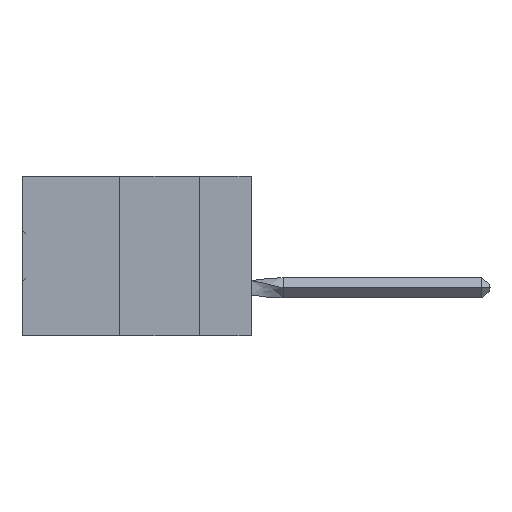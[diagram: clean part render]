
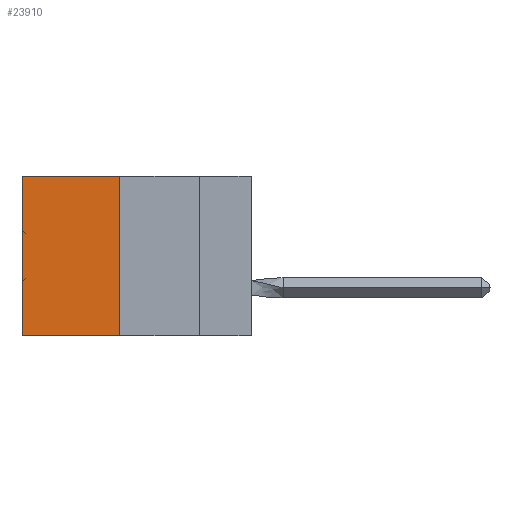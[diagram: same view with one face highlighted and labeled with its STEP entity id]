
A CAD part, left-side view. The second image highlights one B-rep face of the part: STEP entity #23910.
In plain terms, the highlighted planar face has unit normal (-1, 0, 0).
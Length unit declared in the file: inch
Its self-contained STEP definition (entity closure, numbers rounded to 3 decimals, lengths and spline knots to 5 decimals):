
#2695 = CARTESIAN_POINT ( 'NONE',  ( 0.305, 0.413, -0.5 ) ) ;
#3593 = DIRECTION ( 'NONE',  ( 0., 1., 0. ) ) ;
#4007 = CARTESIAN_POINT ( 'NONE',  ( 0.305, 0.413, 0. ) ) ;
#4763 = CARTESIAN_POINT ( 'NONE',  ( 0.305, 0.72, -0.5 ) ) ;
#7627 = CARTESIAN_POINT ( 'NONE',  ( 0.305, 0.413, -0.5 ) ) ;
#9942 = ORIENTED_EDGE ( 'NONE', *, *, #45272, .F. ) ;
#12156 = DIRECTION ( 'NONE',  ( 0., 1., 0. ) ) ;
#12192 = PLANE ( 'NONE',  #33463 ) ;
#13386 = VECTOR ( 'NONE', #12156, 39.37008 ) ;
#17268 = CARTESIAN_POINT ( 'NONE',  ( 0.305, 0.413, -0.5 ) ) ;
#17819 = VERTEX_POINT ( 'NONE', #25723 ) ;
#18130 = FACE_OUTER_BOUND ( 'NONE', #22927, .T. ) ;
#18788 = VECTOR ( 'NONE', #39322, 39.37008 ) ;
#19635 = VERTEX_POINT ( 'NONE', #52158 ) ;
#22927 = EDGE_LOOP ( 'NONE', ( #52261, #9942, #37800, #55808 ) ) ;
#23910 = ADVANCED_FACE ( 'NONE', ( #18130 ), #12192, .F. ) ;
#24987 = EDGE_CURVE ( 'NONE', #19635, #41648, #39858, .T. ) ;
#25723 = CARTESIAN_POINT ( 'NONE',  ( 0.305, 0.72, 0. ) ) ;
#33463 = AXIS2_PLACEMENT_3D ( 'NONE', #38744, #57142, #34438 ) ;
#33806 = EDGE_CURVE ( 'NONE', #17819, #42334, #48794, .T. ) ;
#34438 = DIRECTION ( 'NONE',  ( 0., 0., -1. ) ) ;
#37800 = ORIENTED_EDGE ( 'NONE', *, *, #24987, .F. ) ;
#38744 = CARTESIAN_POINT ( 'NONE',  ( 0.305, 0.413, -0.5 ) ) ;
#39231 = LINE ( 'NONE', #4007, #49724 ) ;
#39322 = DIRECTION ( 'NONE',  ( 0., 0., -1. ) ) ;
#39858 = LINE ( 'NONE', #17268, #18788 ) ;
#40757 = DIRECTION ( 'NONE',  ( 0., 0., -1. ) ) ;
#41648 = VERTEX_POINT ( 'NONE', #2695 ) ;
#42334 = VERTEX_POINT ( 'NONE', #51337 ) ;
#43498 = EDGE_CURVE ( 'NONE', #19635, #17819, #39231, .T. ) ;
#45272 = EDGE_CURVE ( 'NONE', #41648, #42334, #49955, .T. ) ;
#46730 = VECTOR ( 'NONE', #40757, 39.37008 ) ;
#48794 = LINE ( 'NONE', #4763, #46730 ) ;
#49724 = VECTOR ( 'NONE', #3593, 39.37008 ) ;
#49955 = LINE ( 'NONE', #7627, #13386 ) ;
#51337 = CARTESIAN_POINT ( 'NONE',  ( 0.305, 0.72, -0.5 ) ) ;
#52158 = CARTESIAN_POINT ( 'NONE',  ( 0.305, 0.413, 0. ) ) ;
#52261 = ORIENTED_EDGE ( 'NONE', *, *, #33806, .T. ) ;
#55808 = ORIENTED_EDGE ( 'NONE', *, *, #43498, .T. ) ;
#57142 = DIRECTION ( 'NONE',  ( 1., 0., 0. ) ) ;
